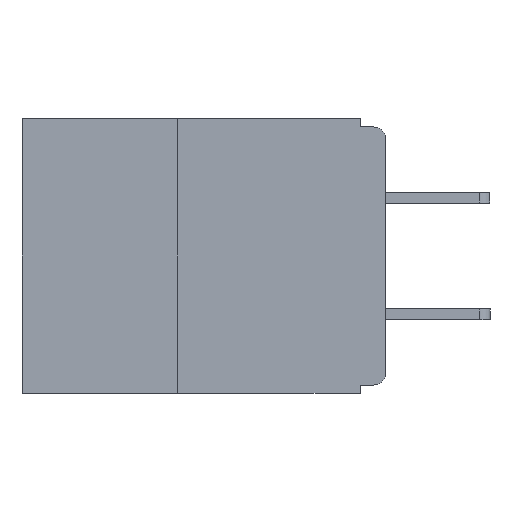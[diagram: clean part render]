
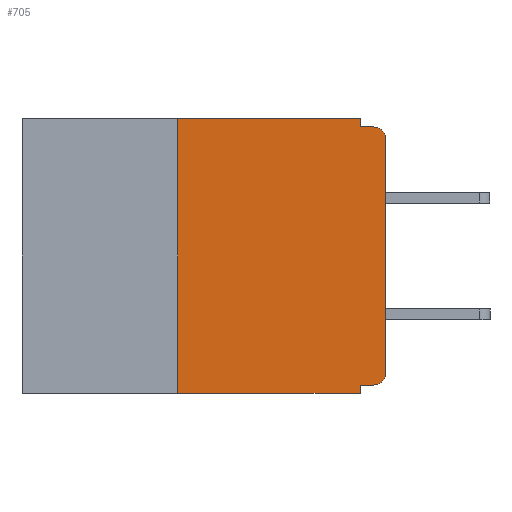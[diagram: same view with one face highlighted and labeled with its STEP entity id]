
A CAD part, left-side view. The second image highlights one B-rep face of the part: STEP entity #705.
In plain terms, the highlighted planar face has unit normal (-1, 0, 0).
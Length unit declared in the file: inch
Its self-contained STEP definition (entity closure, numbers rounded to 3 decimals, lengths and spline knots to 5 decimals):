
#215 = ORIENTED_EDGE ( 'NONE', *, *, #4833, .T. ) ;
#230 = ORIENTED_EDGE ( 'NONE', *, *, #2731, .F. ) ;
#456 = CARTESIAN_POINT ( 'NONE',  ( 0., 0.015, -0.305 ) ) ;
#550 = VERTEX_POINT ( 'NONE', #4387 ) ;
#682 = DIRECTION ( 'NONE',  ( 0., 0., -1. ) ) ;
#705 = ADVANCED_FACE ( 'NONE', ( #16465 ), #7769, .F. ) ;
#756 = CARTESIAN_POINT ( 'NONE',  ( 0., 0.031, -0.33 ) ) ;
#823 = AXIS2_PLACEMENT_3D ( 'NONE', #4115, #2832, #8159 ) ;
#1115 = CARTESIAN_POINT ( 'NONE',  ( 0., 0.031, 0. ) ) ;
#1160 = VECTOR ( 'NONE', #5118, 39.37008 ) ;
#1240 = CIRCLE ( 'NONE', #10887, 0.015 ) ;
#1364 = CARTESIAN_POINT ( 'NONE',  ( 0., 0., 0. ) ) ;
#1491 = VERTEX_POINT ( 'NONE', #9450 ) ;
#2108 = DIRECTION ( 'NONE',  ( 0., 0., -1. ) ) ;
#2250 = ORIENTED_EDGE ( 'NONE', *, *, #14527, .F. ) ;
#2371 = ORIENTED_EDGE ( 'NONE', *, *, #15174, .T. ) ;
#2679 = LINE ( 'NONE', #12479, #1160 ) ;
#2731 = EDGE_CURVE ( 'NONE', #5865, #1491, #11227, .T. ) ;
#2832 = DIRECTION ( 'NONE',  ( 1., 0., 0. ) ) ;
#2924 = VERTEX_POINT ( 'NONE', #5166 ) ;
#3413 = ORIENTED_EDGE ( 'NONE', *, *, #7912, .F. ) ;
#4115 = CARTESIAN_POINT ( 'NONE',  ( 0., 0.437, 0. ) ) ;
#4200 = EDGE_CURVE ( 'NONE', #550, #9497, #1240, .T. ) ;
#4387 = CARTESIAN_POINT ( 'NONE',  ( 0., 0., -0.025 ) ) ;
#4833 = EDGE_CURVE ( 'NONE', #8987, #1491, #7188, .T. ) ;
#4892 = EDGE_LOOP ( 'NONE', ( #15317, #12481, #3413, #5783, #10195, #9536, #215, #230, #2250, #2371 ) ) ;
#5118 = DIRECTION ( 'NONE',  ( 0., 0., -1. ) ) ;
#5166 = CARTESIAN_POINT ( 'NONE',  ( 0., 0.25, 0. ) ) ;
#5775 = LINE ( 'NONE', #15665, #9247 ) ;
#5783 = ORIENTED_EDGE ( 'NONE', *, *, #14130, .F. ) ;
#5804 = EDGE_CURVE ( 'NONE', #8987, #2924, #9514, .T. ) ;
#5819 = LINE ( 'NONE', #1364, #9298 ) ;
#5865 = VERTEX_POINT ( 'NONE', #9550 ) ;
#5932 = LINE ( 'NONE', #15341, #17370 ) ;
#6231 = LINE ( 'NONE', #9635, #9699 ) ;
#7188 = LINE ( 'NONE', #18102, #18621 ) ;
#7769 = PLANE ( 'NONE',  #823 ) ;
#7912 = EDGE_CURVE ( 'NONE', #13105, #9497, #5932, .T. ) ;
#8159 = DIRECTION ( 'NONE',  ( 0., 0., -1. ) ) ;
#8987 = VERTEX_POINT ( 'NONE', #14744 ) ;
#9247 = VECTOR ( 'NONE', #12613, 39.37008 ) ;
#9298 = VECTOR ( 'NONE', #13422, 39.37008 ) ;
#9450 = CARTESIAN_POINT ( 'NONE',  ( 0., 0.031, -0.33 ) ) ;
#9497 = VERTEX_POINT ( 'NONE', #14726 ) ;
#9514 = LINE ( 'NONE', #10883, #12985 ) ;
#9536 = ORIENTED_EDGE ( 'NONE', *, *, #5804, .F. ) ;
#9550 = CARTESIAN_POINT ( 'NONE',  ( 0., 0.031, -0.32 ) ) ;
#9635 = CARTESIAN_POINT ( 'NONE',  ( 0., 0., -0.32 ) ) ;
#9699 = VECTOR ( 'NONE', #11096, 39.37008 ) ;
#10107 = CARTESIAN_POINT ( 'NONE',  ( 0., 0.031, -0.01 ) ) ;
#10195 = ORIENTED_EDGE ( 'NONE', *, *, #14555, .F. ) ;
#10346 = DIRECTION ( 'NONE',  ( -1., 0., 0. ) ) ;
#10814 = DIRECTION ( 'NONE',  ( 0., 0., 1. ) ) ;
#10883 = CARTESIAN_POINT ( 'NONE',  ( 0., 0.25, -0.33 ) ) ;
#10887 = AXIS2_PLACEMENT_3D ( 'NONE', #15385, #10346, #10913 ) ;
#10913 = DIRECTION ( 'NONE',  ( 0., 0., -1. ) ) ;
#11072 = DIRECTION ( 'NONE',  ( -1., 0., 0. ) ) ;
#11096 = DIRECTION ( 'NONE',  ( 0., 1., 0. ) ) ;
#11227 = LINE ( 'NONE', #756, #14758 ) ;
#12479 = CARTESIAN_POINT ( 'NONE',  ( 0., 0.031, 0. ) ) ;
#12481 = ORIENTED_EDGE ( 'NONE', *, *, #4200, .T. ) ;
#12613 = DIRECTION ( 'NONE',  ( 0., -1., 0. ) ) ;
#12782 = AXIS2_PLACEMENT_3D ( 'NONE', #456, #11072, #2108 ) ;
#12974 = CARTESIAN_POINT ( 'NONE',  ( 0., 0.015, -0.32 ) ) ;
#12985 = VECTOR ( 'NONE', #10814, 39.37008 ) ;
#13105 = VERTEX_POINT ( 'NONE', #10107 ) ;
#13248 = EDGE_CURVE ( 'NONE', #15874, #550, #5819, .T. ) ;
#13422 = DIRECTION ( 'NONE',  ( 0., 0., 1. ) ) ;
#14130 = EDGE_CURVE ( 'NONE', #14827, #13105, #2679, .T. ) ;
#14527 = EDGE_CURVE ( 'NONE', #18214, #5865, #6231, .T. ) ;
#14555 = EDGE_CURVE ( 'NONE', #2924, #14827, #5775, .T. ) ;
#14726 = CARTESIAN_POINT ( 'NONE',  ( 0., 0.015, -0.01 ) ) ;
#14744 = CARTESIAN_POINT ( 'NONE',  ( 0., 0.25, -0.33 ) ) ;
#14758 = VECTOR ( 'NONE', #682, 39.37008 ) ;
#14815 = CIRCLE ( 'NONE', #12782, 0.015 ) ;
#14827 = VERTEX_POINT ( 'NONE', #1115 ) ;
#15174 = EDGE_CURVE ( 'NONE', #18214, #15874, #14815, .T. ) ;
#15317 = ORIENTED_EDGE ( 'NONE', *, *, #13248, .T. ) ;
#15341 = CARTESIAN_POINT ( 'NONE',  ( 0., 0., -0.01 ) ) ;
#15385 = CARTESIAN_POINT ( 'NONE',  ( 0., 0.015, -0.025 ) ) ;
#15665 = CARTESIAN_POINT ( 'NONE',  ( 0., 0.437, 0. ) ) ;
#15729 = DIRECTION ( 'NONE',  ( 0., -1., 0. ) ) ;
#15874 = VERTEX_POINT ( 'NONE', #17180 ) ;
#16465 = FACE_OUTER_BOUND ( 'NONE', #4892, .T. ) ;
#17180 = CARTESIAN_POINT ( 'NONE',  ( 0., 0., -0.305 ) ) ;
#17370 = VECTOR ( 'NONE', #15729, 39.37008 ) ;
#17861 = DIRECTION ( 'NONE',  ( 0., -1., 0. ) ) ;
#18102 = CARTESIAN_POINT ( 'NONE',  ( 0., 0.437, -0.33 ) ) ;
#18214 = VERTEX_POINT ( 'NONE', #12974 ) ;
#18621 = VECTOR ( 'NONE', #17861, 39.37008 ) ;
